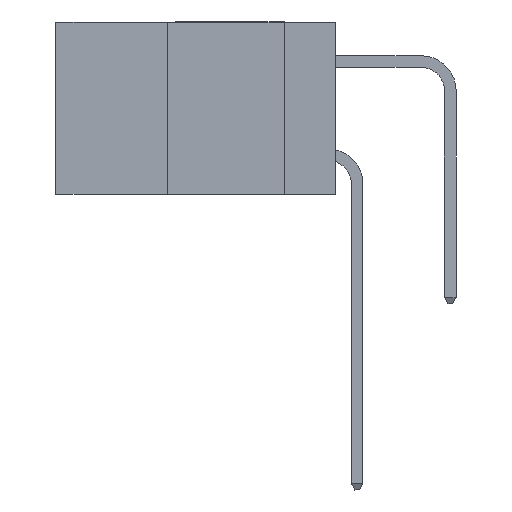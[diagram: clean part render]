
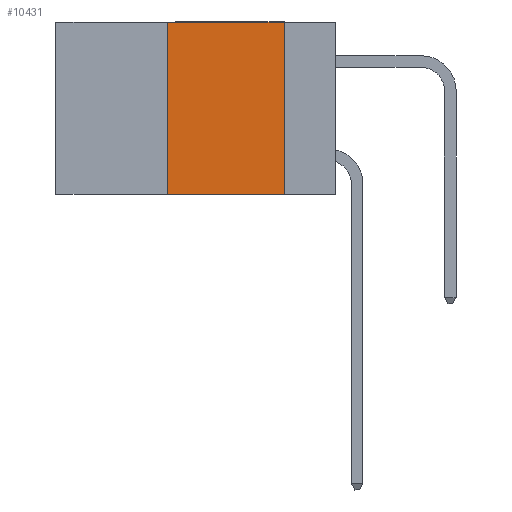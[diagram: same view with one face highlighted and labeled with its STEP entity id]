
A CAD part, left-side view. The second image highlights one B-rep face of the part: STEP entity #10431.
In plain terms, the highlighted planar face has unit normal (-1, 0, 0).
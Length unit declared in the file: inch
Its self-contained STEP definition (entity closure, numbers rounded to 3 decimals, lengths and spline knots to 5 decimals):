
#293 = AXIS2_PLACEMENT_3D ( 'NONE', #9748, #10507, #5844 ) ;
#584 = CARTESIAN_POINT ( 'NONE',  ( 0., 0.11, 0. ) ) ;
#1071 = CARTESIAN_POINT ( 'NONE',  ( 0., 0.6, -0.37 ) ) ;
#1135 = DIRECTION ( 'NONE',  ( 0., -1., 0. ) ) ;
#1748 = LINE ( 'NONE', #1783, #8007 ) ;
#1783 = CARTESIAN_POINT ( 'NONE',  ( 0., 0.6, 0. ) ) ;
#2255 = DIRECTION ( 'NONE',  ( 0., 0., -1. ) ) ;
#2824 = ORIENTED_EDGE ( 'NONE', *, *, #5130, .F. ) ;
#2827 = FACE_OUTER_BOUND ( 'NONE', #6716, .T. ) ;
#2930 = VECTOR ( 'NONE', #2255, 39.37008 ) ;
#3085 = EDGE_CURVE ( 'NONE', #3503, #10174, #3652, .T. ) ;
#3277 = EDGE_CURVE ( 'NONE', #3503, #5231, #6320, .T. ) ;
#3503 = VERTEX_POINT ( 'NONE', #5553 ) ;
#3652 = LINE ( 'NONE', #3952, #9849 ) ;
#3952 = CARTESIAN_POINT ( 'NONE',  ( 0., 0.36, 0. ) ) ;
#4074 = VECTOR ( 'NONE', #1135, 39.37008 ) ;
#4139 = PLANE ( 'NONE',  #293 ) ;
#4622 = CARTESIAN_POINT ( 'NONE',  ( 0., 0.36, 0. ) ) ;
#5130 = EDGE_CURVE ( 'NONE', #10053, #5231, #7444, .T. ) ;
#5231 = VERTEX_POINT ( 'NONE', #9416 ) ;
#5257 = ORIENTED_EDGE ( 'NONE', *, *, #3085, .F. ) ;
#5553 = CARTESIAN_POINT ( 'NONE',  ( 0., 0.36, -0.37 ) ) ;
#5844 = DIRECTION ( 'NONE',  ( 0., 0., -1. ) ) ;
#5853 = DIRECTION ( 'NONE',  ( 0., 0., 1. ) ) ;
#6320 = LINE ( 'NONE', #1071, #4074 ) ;
#6716 = EDGE_LOOP ( 'NONE', ( #2824, #7808, #5257, #8109 ) ) ;
#7444 = LINE ( 'NONE', #584, #2930 ) ;
#7808 = ORIENTED_EDGE ( 'NONE', *, *, #9498, .F. ) ;
#8007 = VECTOR ( 'NONE', #10713, 39.37008 ) ;
#8109 = ORIENTED_EDGE ( 'NONE', *, *, #3277, .T. ) ;
#9416 = CARTESIAN_POINT ( 'NONE',  ( 0., 0.11, -0.37 ) ) ;
#9498 = EDGE_CURVE ( 'NONE', #10174, #10053, #1748, .T. ) ;
#9748 = CARTESIAN_POINT ( 'NONE',  ( 0., 0.6, 0. ) ) ;
#9849 = VECTOR ( 'NONE', #5853, 39.37008 ) ;
#10009 = CARTESIAN_POINT ( 'NONE',  ( 0., 0.11, 0. ) ) ;
#10053 = VERTEX_POINT ( 'NONE', #10009 ) ;
#10174 = VERTEX_POINT ( 'NONE', #4622 ) ;
#10431 = ADVANCED_FACE ( 'NONE', ( #2827 ), #4139, .F. ) ;
#10507 = DIRECTION ( 'NONE',  ( 1., 0., 0. ) ) ;
#10713 = DIRECTION ( 'NONE',  ( 0., -1., 0. ) ) ;
